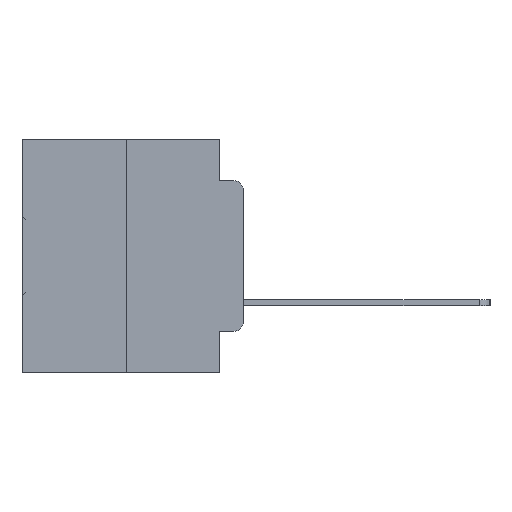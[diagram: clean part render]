
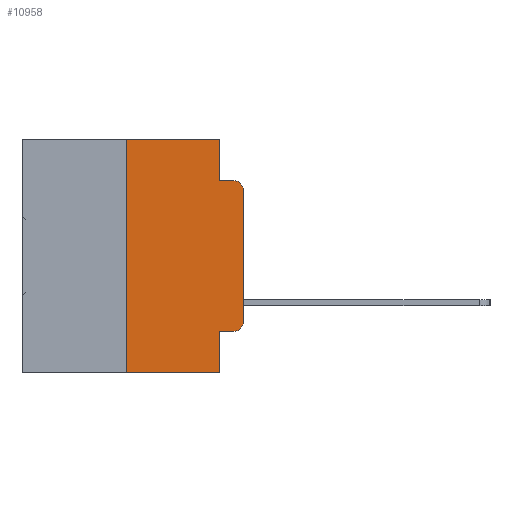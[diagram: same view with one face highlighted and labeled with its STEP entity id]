
A CAD part, left-side view. The second image highlights one B-rep face of the part: STEP entity #10958.
In plain terms, the highlighted planar face has unit normal (-1, 0, 0).
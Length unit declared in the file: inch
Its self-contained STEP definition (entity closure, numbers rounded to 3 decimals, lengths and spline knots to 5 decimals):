
#652 = ORIENTED_EDGE ( 'NONE', *, *, #32672, .T. ) ;
#669 = EDGE_CURVE ( 'NONE', #25439, #4251, #19965, .T. ) ;
#1163 = CARTESIAN_POINT ( 'NONE',  ( 0., 0.051, 0. ) ) ;
#1217 = CARTESIAN_POINT ( 'NONE',  ( 0., 0.051, -0.0885 ) ) ;
#1572 = ORIENTED_EDGE ( 'NONE', *, *, #21564, .F. ) ;
#1907 = AXIS2_PLACEMENT_3D ( 'NONE', #14479, #32968, #17166 ) ;
#2348 = VERTEX_POINT ( 'NONE', #24464 ) ;
#2490 = CARTESIAN_POINT ( 'NONE',  ( 0., 0., -0.3915 ) ) ;
#2884 = EDGE_CURVE ( 'NONE', #23176, #21190, #13766, .T. ) ;
#2927 = CARTESIAN_POINT ( 'NONE',  ( 0., 0.25, 0. ) ) ;
#3293 = CARTESIAN_POINT ( 'NONE',  ( 0., 0.051, -0.4115 ) ) ;
#3459 = VERTEX_POINT ( 'NONE', #9578 ) ;
#3914 = DIRECTION ( 'NONE',  ( 0., 0., -1. ) ) ;
#3959 = CARTESIAN_POINT ( 'NONE',  ( 0., 0.25, -0.5 ) ) ;
#4151 = ORIENTED_EDGE ( 'NONE', *, *, #15224, .F. ) ;
#4209 = DIRECTION ( 'NONE',  ( -1., 0., 0. ) ) ;
#4251 = VERTEX_POINT ( 'NONE', #2490 ) ;
#4581 = EDGE_CURVE ( 'NONE', #25134, #26909, #30647, .T. ) ;
#4705 = CARTESIAN_POINT ( 'NONE',  ( 0., 0.473, -0.5 ) ) ;
#4804 = LINE ( 'NONE', #4705, #17518 ) ;
#5129 = ORIENTED_EDGE ( 'NONE', *, *, #13498, .T. ) ;
#5380 = CARTESIAN_POINT ( 'NONE',  ( 0., 0.02, -0.0885 ) ) ;
#6714 = EDGE_LOOP ( 'NONE', ( #652, #14341, #13955, #1572, #8650, #7417, #24341, #4151, #5129, #10383 ) ) ;
#7057 = CARTESIAN_POINT ( 'NONE',  ( 0., 0.02, -0.4115 ) ) ;
#7126 = VECTOR ( 'NONE', #12121, 39.37008 ) ;
#7323 = FACE_OUTER_BOUND ( 'NONE', #6714, .T. ) ;
#7417 = ORIENTED_EDGE ( 'NONE', *, *, #31113, .F. ) ;
#7586 = CARTESIAN_POINT ( 'NONE',  ( 0., 0.051, 0. ) ) ;
#8012 = LINE ( 'NONE', #9383, #7126 ) ;
#8395 = CIRCLE ( 'NONE', #1907, 0.02 ) ;
#8650 = ORIENTED_EDGE ( 'NONE', *, *, #2884, .F. ) ;
#8916 = AXIS2_PLACEMENT_3D ( 'NONE', #20381, #4209, #23069 ) ;
#9383 = CARTESIAN_POINT ( 'NONE',  ( 0., 0.051, 0. ) ) ;
#9578 = CARTESIAN_POINT ( 'NONE',  ( 0., 0.051, -0.4115 ) ) ;
#9992 = CARTESIAN_POINT ( 'NONE',  ( 0., 0.473, 0. ) ) ;
#10383 = ORIENTED_EDGE ( 'NONE', *, *, #669, .T. ) ;
#10798 = VECTOR ( 'NONE', #18374, 39.37008 ) ;
#10958 = ADVANCED_FACE ( 'NONE', ( #7323 ), #27208, .F. ) ;
#11329 = CARTESIAN_POINT ( 'NONE',  ( 0., 0.473, 0. ) ) ;
#11382 = CARTESIAN_POINT ( 'NONE',  ( 0., 0.25, 0. ) ) ;
#11940 = LINE ( 'NONE', #3293, #16467 ) ;
#12010 = CARTESIAN_POINT ( 'NONE',  ( 0., 0.051, -0.0885 ) ) ;
#12121 = DIRECTION ( 'NONE',  ( 0., 0., -1. ) ) ;
#12183 = LINE ( 'NONE', #2927, #18390 ) ;
#13498 = EDGE_CURVE ( 'NONE', #3459, #25439, #11940, .T. ) ;
#13766 = LINE ( 'NONE', #9992, #33192 ) ;
#13955 = ORIENTED_EDGE ( 'NONE', *, *, #4581, .F. ) ;
#14341 = ORIENTED_EDGE ( 'NONE', *, *, #22113, .T. ) ;
#14479 = CARTESIAN_POINT ( 'NONE',  ( 0., 0.02, -0.1085 ) ) ;
#14596 = VERTEX_POINT ( 'NONE', #3959 ) ;
#14641 = DIRECTION ( 'NONE',  ( 0., -1., 0. ) ) ;
#15044 = CARTESIAN_POINT ( 'NONE',  ( 0., 0., -0.1085 ) ) ;
#15224 = EDGE_CURVE ( 'NONE', #3459, #2348, #17681, .T. ) ;
#16467 = VECTOR ( 'NONE', #22059, 39.37008 ) ;
#16599 = VECTOR ( 'NONE', #14641, 39.37008 ) ;
#16647 = DIRECTION ( 'NONE',  ( 0., 0., -1. ) ) ;
#16846 = VECTOR ( 'NONE', #3914, 39.37008 ) ;
#17166 = DIRECTION ( 'NONE',  ( 0., 0., -1. ) ) ;
#17518 = VECTOR ( 'NONE', #20973, 39.37008 ) ;
#17681 = LINE ( 'NONE', #1163, #16846 ) ;
#17837 = LINE ( 'NONE', #23689, #10798 ) ;
#18374 = DIRECTION ( 'NONE',  ( 0., 0., 1. ) ) ;
#18390 = VECTOR ( 'NONE', #24479, 39.37008 ) ;
#19965 = CIRCLE ( 'NONE', #8916, 0.02 ) ;
#20381 = CARTESIAN_POINT ( 'NONE',  ( 0., 0.02, -0.3915 ) ) ;
#20529 = DIRECTION ( 'NONE',  ( 0., -1., 0. ) ) ;
#20953 = AXIS2_PLACEMENT_3D ( 'NONE', #11329, #32472, #16647 ) ;
#20973 = DIRECTION ( 'NONE',  ( 0., -1., 0. ) ) ;
#21190 = VERTEX_POINT ( 'NONE', #7586 ) ;
#21564 = EDGE_CURVE ( 'NONE', #21190, #25134, #8012, .T. ) ;
#22059 = DIRECTION ( 'NONE',  ( 0., -1., 0. ) ) ;
#22113 = EDGE_CURVE ( 'NONE', #28979, #26909, #8395, .T. ) ;
#23069 = DIRECTION ( 'NONE',  ( 0., 0., -1. ) ) ;
#23176 = VERTEX_POINT ( 'NONE', #11382 ) ;
#23689 = CARTESIAN_POINT ( 'NONE',  ( 0., 0., 0. ) ) ;
#24341 = ORIENTED_EDGE ( 'NONE', *, *, #31571, .T. ) ;
#24464 = CARTESIAN_POINT ( 'NONE',  ( 0., 0.051, -0.5 ) ) ;
#24479 = DIRECTION ( 'NONE',  ( 0., 0., 1. ) ) ;
#25134 = VERTEX_POINT ( 'NONE', #1217 ) ;
#25439 = VERTEX_POINT ( 'NONE', #7057 ) ;
#26909 = VERTEX_POINT ( 'NONE', #5380 ) ;
#27208 = PLANE ( 'NONE',  #20953 ) ;
#28979 = VERTEX_POINT ( 'NONE', #15044 ) ;
#30647 = LINE ( 'NONE', #12010, #16599 ) ;
#31113 = EDGE_CURVE ( 'NONE', #14596, #23176, #12183, .T. ) ;
#31571 = EDGE_CURVE ( 'NONE', #14596, #2348, #4804, .T. ) ;
#32472 = DIRECTION ( 'NONE',  ( 1., 0., 0. ) ) ;
#32672 = EDGE_CURVE ( 'NONE', #4251, #28979, #17837, .T. ) ;
#32968 = DIRECTION ( 'NONE',  ( -1., 0., 0. ) ) ;
#33192 = VECTOR ( 'NONE', #20529, 39.37008 ) ;
